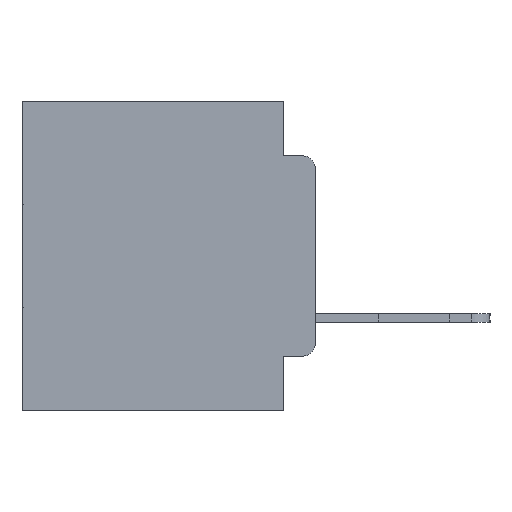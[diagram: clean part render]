
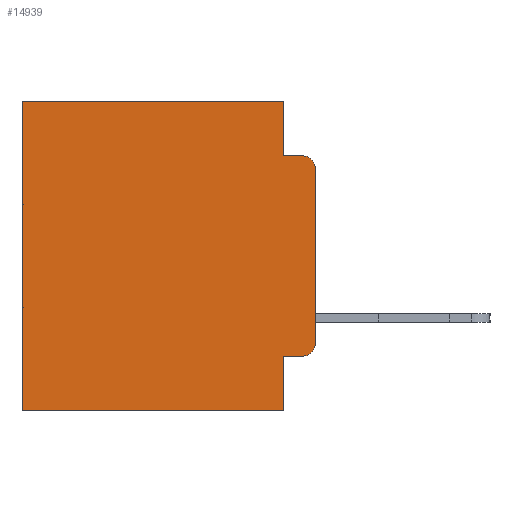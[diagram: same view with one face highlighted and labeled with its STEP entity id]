
A CAD part, left-side view. The second image highlights one B-rep face of the part: STEP entity #14939.
In plain terms, the highlighted planar face has unit normal (-1, 0, 0).
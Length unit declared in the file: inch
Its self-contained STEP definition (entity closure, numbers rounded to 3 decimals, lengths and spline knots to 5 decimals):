
#517 = VECTOR ( 'NONE', #13454, 39.37008 ) ;
#792 = LINE ( 'NONE', #30303, #12660 ) ;
#889 = CARTESIAN_POINT ( 'NONE',  ( 0.298, 0.02, -0.0885 ) ) ;
#965 = EDGE_CURVE ( 'NONE', #15973, #21844, #24708, .T. ) ;
#1156 = EDGE_CURVE ( 'NONE', #13811, #6012, #792, .T. ) ;
#1240 = LINE ( 'NONE', #15845, #517 ) ;
#1548 = ORIENTED_EDGE ( 'NONE', *, *, #1156, .F. ) ;
#2036 = VECTOR ( 'NONE', #19380, 39.37008 ) ;
#2114 = EDGE_CURVE ( 'NONE', #12101, #5935, #28210, .T. ) ;
#2351 = AXIS2_PLACEMENT_3D ( 'NONE', #13689, #29877, #16083 ) ;
#2616 = AXIS2_PLACEMENT_3D ( 'NONE', #4689, #4631, #4312 ) ;
#3403 = LINE ( 'NONE', #9114, #15371 ) ;
#3664 = EDGE_CURVE ( 'NONE', #21844, #19129, #22605, .T. ) ;
#3725 = DIRECTION ( 'NONE',  ( 0., -1., 0. ) ) ;
#4129 = ORIENTED_EDGE ( 'NONE', *, *, #9307, .F. ) ;
#4312 = DIRECTION ( 'NONE',  ( 0., 0., -1. ) ) ;
#4440 = PLANE ( 'NONE',  #20124 ) ;
#4631 = DIRECTION ( 'NONE',  ( -1., 0., 0. ) ) ;
#4689 = CARTESIAN_POINT ( 'NONE',  ( 0.298, 0.02, -0.3915 ) ) ;
#4977 = CIRCLE ( 'NONE', #2351, 0.02 ) ;
#5935 = VERTEX_POINT ( 'NONE', #23917 ) ;
#5972 = VECTOR ( 'NONE', #28654, 39.37008 ) ;
#6012 = VERTEX_POINT ( 'NONE', #11532 ) ;
#6474 = ORIENTED_EDGE ( 'NONE', *, *, #29545, .F. ) ;
#6846 = VECTOR ( 'NONE', #3725, 39.37008 ) ;
#7297 = CARTESIAN_POINT ( 'NONE',  ( 0.298, 0.051, 0. ) ) ;
#7531 = ORIENTED_EDGE ( 'NONE', *, *, #24231, .F. ) ;
#8215 = CARTESIAN_POINT ( 'NONE',  ( 0.298, 0., -0.1085 ) ) ;
#8252 = ORIENTED_EDGE ( 'NONE', *, *, #8365, .T. ) ;
#8294 = EDGE_CURVE ( 'NONE', #15973, #12313, #29138, .T. ) ;
#8365 = EDGE_CURVE ( 'NONE', #13811, #12101, #20915, .T. ) ;
#8727 = EDGE_CURVE ( 'NONE', #13388, #20829, #4977, .T. ) ;
#9114 = CARTESIAN_POINT ( 'NONE',  ( 0.298, 0., -0.5 ) ) ;
#9256 = DIRECTION ( 'NONE',  ( 0., 0., -1. ) ) ;
#9307 = EDGE_CURVE ( 'NONE', #13388, #5935, #1240, .T. ) ;
#9656 = CARTESIAN_POINT ( 'NONE',  ( 0.298, 0.473, 0. ) ) ;
#9744 = CARTESIAN_POINT ( 'NONE',  ( 0.298, 0.051, -0.4115 ) ) ;
#9842 = CARTESIAN_POINT ( 'NONE',  ( 0.298, 0.051, -0.0885 ) ) ;
#10114 = VECTOR ( 'NONE', #30121, 39.37008 ) ;
#11509 = DIRECTION ( 'NONE',  ( 0., 1., 0. ) ) ;
#11532 = CARTESIAN_POINT ( 'NONE',  ( 0.298, 0.051, -0.5 ) ) ;
#12101 = VERTEX_POINT ( 'NONE', #18337 ) ;
#12313 = VERTEX_POINT ( 'NONE', #9842 ) ;
#12660 = VECTOR ( 'NONE', #14901, 39.37008 ) ;
#13021 = CARTESIAN_POINT ( 'NONE',  ( 0.298, 0.473, -0.5 ) ) ;
#13388 = VERTEX_POINT ( 'NONE', #8215 ) ;
#13454 = DIRECTION ( 'NONE',  ( 0., 0., -1. ) ) ;
#13689 = CARTESIAN_POINT ( 'NONE',  ( 0.298, 0.02, -0.1085 ) ) ;
#13811 = VERTEX_POINT ( 'NONE', #9744 ) ;
#13838 = ORIENTED_EDGE ( 'NONE', *, *, #3664, .T. ) ;
#14664 = CARTESIAN_POINT ( 'NONE',  ( 0.298, 0.051, -0.4115 ) ) ;
#14901 = DIRECTION ( 'NONE',  ( 0., 0., -1. ) ) ;
#14939 = ADVANCED_FACE ( 'NONE', ( #21750 ), #4440, .F. ) ;
#15371 = VECTOR ( 'NONE', #11509, 39.37008 ) ;
#15845 = CARTESIAN_POINT ( 'NONE',  ( 0.298, 0., 0. ) ) ;
#15864 = CARTESIAN_POINT ( 'NONE',  ( 0.298, 0., 0. ) ) ;
#15973 = VERTEX_POINT ( 'NONE', #21790 ) ;
#16083 = DIRECTION ( 'NONE',  ( 0., 0., -1. ) ) ;
#16936 = VECTOR ( 'NONE', #19078, 39.37008 ) ;
#17941 = LINE ( 'NONE', #24939, #6846 ) ;
#18337 = CARTESIAN_POINT ( 'NONE',  ( 0.298, 0.02, -0.4115 ) ) ;
#19078 = DIRECTION ( 'NONE',  ( 0., 0., -1. ) ) ;
#19129 = VERTEX_POINT ( 'NONE', #13021 ) ;
#19380 = DIRECTION ( 'NONE',  ( 0., -1., 0. ) ) ;
#20124 = AXIS2_PLACEMENT_3D ( 'NONE', #21001, #23320, #9256 ) ;
#20829 = VERTEX_POINT ( 'NONE', #889 ) ;
#20915 = LINE ( 'NONE', #14664, #2036 ) ;
#21001 = CARTESIAN_POINT ( 'NONE',  ( 0.298, 0., 0. ) ) ;
#21204 = ORIENTED_EDGE ( 'NONE', *, *, #8727, .T. ) ;
#21750 = FACE_OUTER_BOUND ( 'NONE', #27757, .T. ) ;
#21790 = CARTESIAN_POINT ( 'NONE',  ( 0.298, 0.051, 0. ) ) ;
#21844 = VERTEX_POINT ( 'NONE', #9656 ) ;
#22605 = LINE ( 'NONE', #22676, #10114 ) ;
#22676 = CARTESIAN_POINT ( 'NONE',  ( 0.298, 0.473, 0. ) ) ;
#23320 = DIRECTION ( 'NONE',  ( 1., 0., 0. ) ) ;
#23917 = CARTESIAN_POINT ( 'NONE',  ( 0.298, 0., -0.3915 ) ) ;
#24231 = EDGE_CURVE ( 'NONE', #6012, #19129, #3403, .T. ) ;
#24696 = ORIENTED_EDGE ( 'NONE', *, *, #8294, .F. ) ;
#24708 = LINE ( 'NONE', #15864, #5972 ) ;
#24729 = ORIENTED_EDGE ( 'NONE', *, *, #965, .T. ) ;
#24939 = CARTESIAN_POINT ( 'NONE',  ( 0.298, 0.051, -0.0885 ) ) ;
#27757 = EDGE_LOOP ( 'NONE', ( #4129, #21204, #6474, #24696, #24729, #13838, #7531, #1548, #8252, #27943 ) ) ;
#27943 = ORIENTED_EDGE ( 'NONE', *, *, #2114, .T. ) ;
#28210 = CIRCLE ( 'NONE', #2616, 0.02 ) ;
#28654 = DIRECTION ( 'NONE',  ( 0., 1., 0. ) ) ;
#29138 = LINE ( 'NONE', #7297, #16936 ) ;
#29545 = EDGE_CURVE ( 'NONE', #12313, #20829, #17941, .T. ) ;
#29877 = DIRECTION ( 'NONE',  ( -1., 0., 0. ) ) ;
#30121 = DIRECTION ( 'NONE',  ( 0., 0., -1. ) ) ;
#30303 = CARTESIAN_POINT ( 'NONE',  ( 0.298, 0.051, 0. ) ) ;
